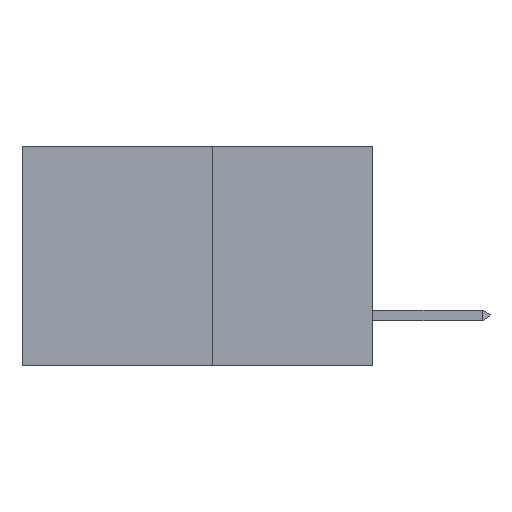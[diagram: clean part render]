
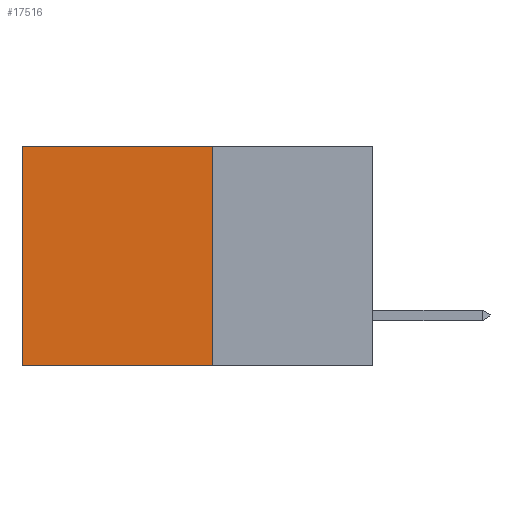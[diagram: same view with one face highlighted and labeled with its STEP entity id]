
A CAD part, left-side view. The second image highlights one B-rep face of the part: STEP entity #17516.
In plain terms, the highlighted planar face has unit normal (-1, 0, 0).
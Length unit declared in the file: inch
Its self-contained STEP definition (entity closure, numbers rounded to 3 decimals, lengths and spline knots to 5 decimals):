
#1477 = EDGE_CURVE ( 'NONE', #14434, #26723, #2621, .T. ) ;
#1897 = ORIENTED_EDGE ( 'NONE', *, *, #1477, .F. ) ;
#2073 = CARTESIAN_POINT ( 'NONE',  ( 0.277, 0.27, 0. ) ) ;
#2092 = DIRECTION ( 'NONE',  ( 0., 1., 0. ) ) ;
#2621 = LINE ( 'NONE', #20805, #21134 ) ;
#2944 = VERTEX_POINT ( 'NONE', #2073 ) ;
#3180 = CARTESIAN_POINT ( 'NONE',  ( 0.277, 0.27, -0.37 ) ) ;
#7119 = LINE ( 'NONE', #26994, #17207 ) ;
#9421 = VERTEX_POINT ( 'NONE', #25417 ) ;
#10056 = CARTESIAN_POINT ( 'NONE',  ( 0.277, 0.27, 0. ) ) ;
#11492 = LINE ( 'NONE', #10056, #16575 ) ;
#11636 = LINE ( 'NONE', #16579, #27446 ) ;
#11674 = ORIENTED_EDGE ( 'NONE', *, *, #13433, .T. ) ;
#12740 = CARTESIAN_POINT ( 'NONE',  ( 0.277, 0.27, -0.37 ) ) ;
#12792 = ORIENTED_EDGE ( 'NONE', *, *, #20753, .T. ) ;
#13369 = FACE_OUTER_BOUND ( 'NONE', #14003, .T. ) ;
#13433 = EDGE_CURVE ( 'NONE', #9421, #26723, #11636, .T. ) ;
#14003 = EDGE_LOOP ( 'NONE', ( #11674, #1897, #21896, #12792 ) ) ;
#14099 = DIRECTION ( 'NONE',  ( 0., 0., -1. ) ) ;
#14434 = VERTEX_POINT ( 'NONE', #3180 ) ;
#14488 = CARTESIAN_POINT ( 'NONE',  ( 0.277, 0.59, -0.37 ) ) ;
#14935 = DIRECTION ( 'NONE',  ( 0., 0., -1. ) ) ;
#15235 = EDGE_CURVE ( 'NONE', #2944, #14434, #7119, .T. ) ;
#16351 = DIRECTION ( 'NONE',  ( 1., 0., 0. ) ) ;
#16575 = VECTOR ( 'NONE', #20936, 39.37008 ) ;
#16579 = CARTESIAN_POINT ( 'NONE',  ( 0.277, 0.59, -0.37 ) ) ;
#17207 = VECTOR ( 'NONE', #14099, 39.37008 ) ;
#17516 = ADVANCED_FACE ( 'NONE', ( #13369 ), #21342, .F. ) ;
#18731 = DIRECTION ( 'NONE',  ( 0., 0., -1. ) ) ;
#19727 = AXIS2_PLACEMENT_3D ( 'NONE', #12740, #16351, #14935 ) ;
#20753 = EDGE_CURVE ( 'NONE', #2944, #9421, #11492, .T. ) ;
#20805 = CARTESIAN_POINT ( 'NONE',  ( 0.277, 0.27, -0.37 ) ) ;
#20936 = DIRECTION ( 'NONE',  ( 0., 1., 0. ) ) ;
#21134 = VECTOR ( 'NONE', #2092, 39.37008 ) ;
#21342 = PLANE ( 'NONE',  #19727 ) ;
#21896 = ORIENTED_EDGE ( 'NONE', *, *, #15235, .F. ) ;
#25417 = CARTESIAN_POINT ( 'NONE',  ( 0.277, 0.59, 0. ) ) ;
#26723 = VERTEX_POINT ( 'NONE', #14488 ) ;
#26994 = CARTESIAN_POINT ( 'NONE',  ( 0.277, 0.27, -0.37 ) ) ;
#27446 = VECTOR ( 'NONE', #18731, 39.37008 ) ;
